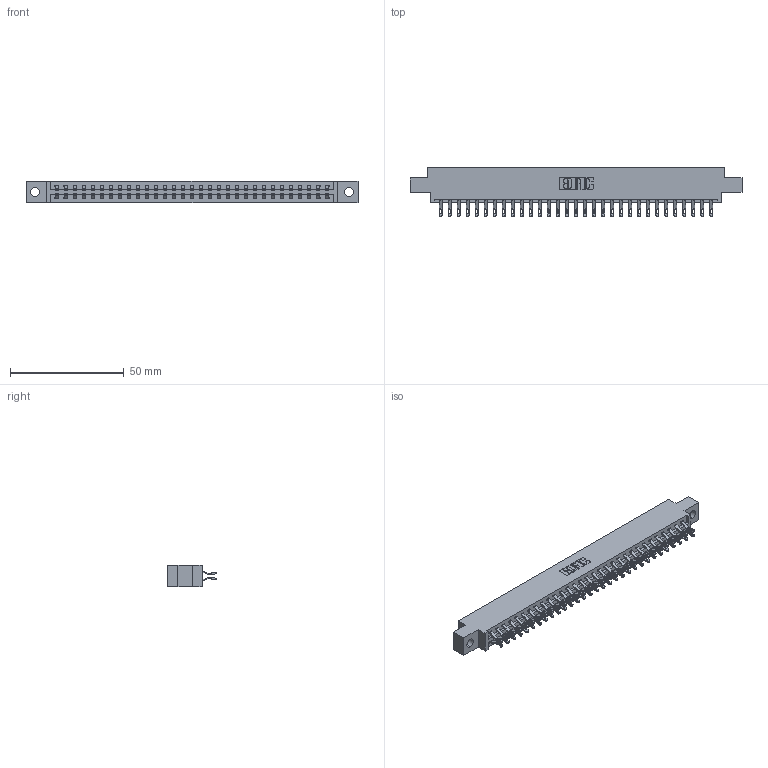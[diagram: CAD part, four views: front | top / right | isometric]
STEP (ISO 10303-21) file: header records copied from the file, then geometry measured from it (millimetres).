
FILE_DESCRIPTION (( 'STEP AP203' ), '1' );
FILE_NAME ('337-062-555-804.STEP', '2018-08-11T04:37:22', ( '' ), ( '' ), 'SwSTEP 2.0', 'SolidWorks 2016', '' );
FILE_SCHEMA (( 'CONFIG_CONTROL_DESIGN' ));
Length unit declared in the file: inch
Products named in the file (3): 345-292-001_555 Tail; 337-062-555-804; 337 Part_0.170 Offset - 0.156 Dia-TH
Assembly tree (63 placements, depth 2):
  337-062-555-804
    337 Part_0.170 Offset - 0.156 Dia-TH
    345-292-001_555 Tail  x62
Bounding box: 145.85 x 21.47 x 9.4 mm (x, y, z)
Volume: 15198.5 mm3; surface area: 17658.1 mm2
Topology: 63 solids, 63 shells, 3838 faces, 12041 edges, 8026 vertices
Faces by surface type: plane 2306, cylinder 1532
Entity records: 25919 total; most frequent: CARTESIAN_POINT 4412, ORIENTED_EDGE 4318, DIRECTION 3743, EDGE_CURVE 2159, VECTOR 2011, LINE 2011, VERTEX_POINT 1438, AXIS2_PLACEMENT_3D 866
